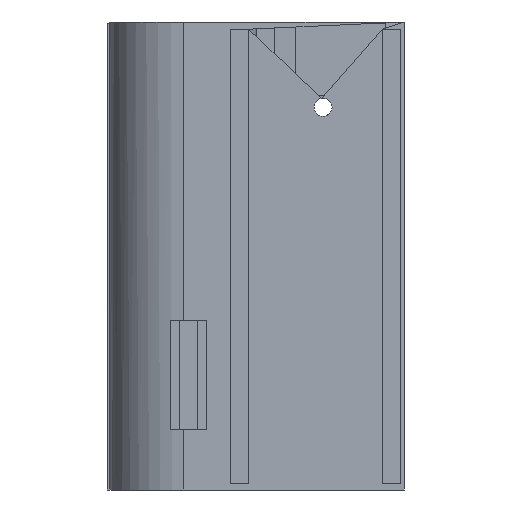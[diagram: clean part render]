
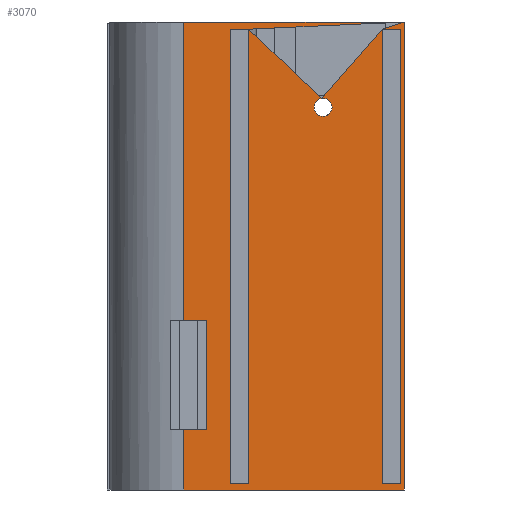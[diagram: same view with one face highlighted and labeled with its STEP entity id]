
A CAD part, left-side view. The second image highlights one B-rep face of the part: STEP entity #3070.
In plain terms, the highlighted planar face has unit normal (-1, 0, 0).
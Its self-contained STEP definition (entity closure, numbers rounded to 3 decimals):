
#5 = DIRECTION ( 'NONE',  ( 0., 0., -1. ) ) ;
#23 = ORIENTED_EDGE ( 'NONE', *, *, #3715, .T. ) ;
#29 = EDGE_CURVE ( 'NONE', #139, #4762, #4374, .T. ) ;
#71 = AXIS2_PLACEMENT_3D ( 'NONE', #1782, #1324, #1346 ) ;
#129 = LINE ( 'NONE', #1166, #960 ) ;
#139 = VERTEX_POINT ( 'NONE', #4965 ) ;
#177 = EDGE_LOOP ( 'NONE', ( #330, #702, #4123, #989 ) ) ;
#210 = EDGE_CURVE ( 'NONE', #4336, #4336, #4398, .T. ) ;
#241 = EDGE_CURVE ( 'NONE', #5273, #1962, #3889, .T. ) ;
#316 = VECTOR ( 'NONE', #2733, 1000. ) ;
#322 = CARTESIAN_POINT ( 'NONE',  ( -13., 25.767, -1. ) ) ;
#330 = ORIENTED_EDGE ( 'NONE', *, *, #569, .T. ) ;
#339 = CARTESIAN_POINT ( 'NONE',  ( -13., -10.668, 76.189 ) ) ;
#361 = DIRECTION ( 'NONE',  ( 0., -1., 0. ) ) ;
#369 = EDGE_CURVE ( 'NONE', #4762, #3531, #3568, .T. ) ;
#400 = EDGE_CURVE ( 'NONE', #467, #139, #3026, .T. ) ;
#467 = VERTEX_POINT ( 'NONE', #1895 ) ;
#504 = FACE_BOUND ( 'NONE', #1764, .T. ) ;
#536 = EDGE_CURVE ( 'NONE', #4986, #589, #129, .T. ) ;
#569 = EDGE_CURVE ( 'NONE', #2528, #1590, #4109, .T. ) ;
#589 = VERTEX_POINT ( 'NONE', #339 ) ;
#626 = DIRECTION ( 'NONE',  ( 0., 1., 0. ) ) ;
#669 = CARTESIAN_POINT ( 'NONE',  ( -13., -10.668, -1. ) ) ;
#702 = ORIENTED_EDGE ( 'NONE', *, *, #4699, .T. ) ;
#758 = CARTESIAN_POINT ( 'NONE',  ( -13., 25.767, 76.189 ) ) ;
#786 = CARTESIAN_POINT ( 'NONE',  ( -13., -10., 0. ) ) ;
#866 = CARTESIAN_POINT ( 'NONE',  ( -13., 21.9, 9. ) ) ;
#931 = CARTESIAN_POINT ( 'NONE',  ( -13., 21.9, 9. ) ) ;
#960 = VECTOR ( 'NONE', #1559, 1000. ) ;
#989 = ORIENTED_EDGE ( 'NONE', *, *, #3333, .T. ) ;
#1023 = VERTEX_POINT ( 'NONE', #758 ) ;
#1067 = VECTOR ( 'NONE', #1955, 1000. ) ;
#1096 = EDGE_LOOP ( 'NONE', ( #4860, #1400, #1157, #2286, #1209, #4950, #2393, #23 ) ) ;
#1124 = CARTESIAN_POINT ( 'NONE',  ( -13., 25.767, -1. ) ) ;
#1134 = CARTESIAN_POINT ( 'NONE',  ( -13., 25.767, -1. ) ) ;
#1154 = CARTESIAN_POINT ( 'NONE',  ( -13., 27.9, 27. ) ) ;
#1157 = ORIENTED_EDGE ( 'NONE', *, *, #3190, .T. ) ;
#1166 = CARTESIAN_POINT ( 'NONE',  ( -13., -10.668, -1. ) ) ;
#1205 = FACE_BOUND ( 'NONE', #177, .T. ) ;
#1209 = ORIENTED_EDGE ( 'NONE', *, *, #5067, .F. ) ;
#1219 = VECTOR ( 'NONE', #2648, 1000. ) ;
#1324 = DIRECTION ( 'NONE',  ( 1., 0., 0. ) ) ;
#1342 = PLANE ( 'NONE',  #2740 ) ;
#1346 = DIRECTION ( 'NONE',  ( 0., 1., 0. ) ) ;
#1400 = ORIENTED_EDGE ( 'NONE', *, *, #3306, .T. ) ;
#1415 = CARTESIAN_POINT ( 'NONE',  ( -13., 21.9, 27. ) ) ;
#1431 = VERTEX_POINT ( 'NONE', #322 ) ;
#1435 = CARTESIAN_POINT ( 'NONE',  ( -13., 18., 75. ) ) ;
#1449 = LINE ( 'NONE', #2551, #4335 ) ;
#1476 = EDGE_LOOP ( 'NONE', ( #4700, #1900, #1536, #1498 ) ) ;
#1490 = VERTEX_POINT ( 'NONE', #3621 ) ;
#1493 = VERTEX_POINT ( 'NONE', #2443 ) ;
#1498 = ORIENTED_EDGE ( 'NONE', *, *, #5166, .T. ) ;
#1505 = ORIENTED_EDGE ( 'NONE', *, *, #210, .T. ) ;
#1511 = EDGE_CURVE ( 'NONE', #1639, #1493, #5157, .T. ) ;
#1536 = ORIENTED_EDGE ( 'NONE', *, *, #369, .T. ) ;
#1559 = DIRECTION ( 'NONE',  ( 0., 0., 1. ) ) ;
#1590 = VERTEX_POINT ( 'NONE', #3296 ) ;
#1639 = VERTEX_POINT ( 'NONE', #4127 ) ;
#1708 = VECTOR ( 'NONE', #4285, 1000. ) ;
#1764 = EDGE_LOOP ( 'NONE', ( #1505 ) ) ;
#1782 = CARTESIAN_POINT ( 'NONE',  ( -13., 2.757, 62.126 ) ) ;
#1864 = VECTOR ( 'NONE', #4481, 1000. ) ;
#1895 = CARTESIAN_POINT ( 'NONE',  ( -13., 15., 0. ) ) ;
#1900 = ORIENTED_EDGE ( 'NONE', *, *, #29, .T. ) ;
#1955 = DIRECTION ( 'NONE',  ( 0., 0., 1. ) ) ;
#1962 = VERTEX_POINT ( 'NONE', #2776 ) ;
#2050 = LINE ( 'NONE', #1154, #1864 ) ;
#2109 = LINE ( 'NONE', #3135, #2825 ) ;
#2285 = CARTESIAN_POINT ( 'NONE',  ( -13., 15., 0. ) ) ;
#2286 = ORIENTED_EDGE ( 'NONE', *, *, #241, .T. ) ;
#2292 = LINE ( 'NONE', #4842, #4209 ) ;
#2372 = LINE ( 'NONE', #786, #2635 ) ;
#2380 = CARTESIAN_POINT ( 'NONE',  ( -13., 18., 0. ) ) ;
#2393 = ORIENTED_EDGE ( 'NONE', *, *, #536, .T. ) ;
#2414 = CARTESIAN_POINT ( 'NONE',  ( -13., 45.608, -1. ) ) ;
#2430 = LINE ( 'NONE', #2414, #2834 ) ;
#2443 = CARTESIAN_POINT ( 'NONE',  ( -13., -10., 0. ) ) ;
#2499 = DIRECTION ( 'NONE',  ( 0., -1., 0. ) ) ;
#2528 = VERTEX_POINT ( 'NONE', #4625 ) ;
#2551 = CARTESIAN_POINT ( 'NONE',  ( -13., -7., 75. ) ) ;
#2635 = VECTOR ( 'NONE', #4028, 1000. ) ;
#2648 = DIRECTION ( 'NONE',  ( 0., 1., 0. ) ) ;
#2698 = VECTOR ( 'NONE', #3248, 1000. ) ;
#2733 = DIRECTION ( 'NONE',  ( 0., 0., -1. ) ) ;
#2740 = AXIS2_PLACEMENT_3D ( 'NONE', #3395, #3783, #4595 ) ;
#2776 = CARTESIAN_POINT ( 'NONE',  ( -13., 25.767, 9. ) ) ;
#2825 = VECTOR ( 'NONE', #626, 1000. ) ;
#2834 = VECTOR ( 'NONE', #361, 1000. ) ;
#2890 = VECTOR ( 'NONE', #3910, 1000. ) ;
#2907 = LINE ( 'NONE', #1415, #5278 ) ;
#2914 = EDGE_CURVE ( 'NONE', #1023, #1490, #4107, .T. ) ;
#3026 = LINE ( 'NONE', #2285, #1219 ) ;
#3070 = ADVANCED_FACE ( 'NONE', ( #3658, #4849, #1205, #504 ), #1342, .T. ) ;
#3135 = CARTESIAN_POINT ( 'NONE',  ( -13., 15.471, 76.189 ) ) ;
#3190 = EDGE_CURVE ( 'NONE', #4493, #5273, #2907, .T. ) ;
#3213 = DIRECTION ( 'NONE',  ( 0., 0., 1. ) ) ;
#3232 = VECTOR ( 'NONE', #3213, 1000. ) ;
#3248 = DIRECTION ( 'NONE',  ( 0., 0., -1. ) ) ;
#3296 = CARTESIAN_POINT ( 'NONE',  ( -13., -7., 75. ) ) ;
#3297 = VECTOR ( 'NONE', #4428, 1000. ) ;
#3306 = EDGE_CURVE ( 'NONE', #1490, #4493, #2050, .T. ) ;
#3315 = EDGE_CURVE ( 'NONE', #1431, #4986, #2430, .T. ) ;
#3333 = EDGE_CURVE ( 'NONE', #1493, #2528, #2372, .T. ) ;
#3395 = CARTESIAN_POINT ( 'NONE',  ( -13., -10.668, -1. ) ) ;
#3450 = CARTESIAN_POINT ( 'NONE',  ( -13., 15., 75. ) ) ;
#3531 = VERTEX_POINT ( 'NONE', #3450 ) ;
#3568 = LINE ( 'NONE', #1435, #2890 ) ;
#3619 = CARTESIAN_POINT ( 'NONE',  ( -13., -7., 0. ) ) ;
#3621 = CARTESIAN_POINT ( 'NONE',  ( -13., 25.767, 27. ) ) ;
#3658 = FACE_BOUND ( 'NONE', #1476, .T. ) ;
#3700 = LINE ( 'NONE', #1124, #1067 ) ;
#3715 = EDGE_CURVE ( 'NONE', #589, #1023, #2109, .T. ) ;
#3783 = DIRECTION ( 'NONE',  ( -1., 0., 0. ) ) ;
#3813 = CARTESIAN_POINT ( 'NONE',  ( -13., 18., 75. ) ) ;
#3889 = LINE ( 'NONE', #931, #1708 ) ;
#3910 = DIRECTION ( 'NONE',  ( 0., -1., 0. ) ) ;
#4028 = DIRECTION ( 'NONE',  ( 0., 1., 0. ) ) ;
#4107 = LINE ( 'NONE', #1134, #316 ) ;
#4109 = LINE ( 'NONE', #3619, #3232 ) ;
#4123 = ORIENTED_EDGE ( 'NONE', *, *, #1511, .T. ) ;
#4127 = CARTESIAN_POINT ( 'NONE',  ( -13., -10., 75. ) ) ;
#4209 = VECTOR ( 'NONE', #5, 1000. ) ;
#4282 = DIRECTION ( 'NONE',  ( 0., 0., -1. ) ) ;
#4285 = DIRECTION ( 'NONE',  ( 0., 1., 0. ) ) ;
#4335 = VECTOR ( 'NONE', #2499, 1000. ) ;
#4336 = VERTEX_POINT ( 'NONE', #4553 ) ;
#4374 = LINE ( 'NONE', #2380, #3297 ) ;
#4398 = CIRCLE ( 'NONE', #71, 1.484 ) ;
#4428 = DIRECTION ( 'NONE',  ( 0., 0., 1. ) ) ;
#4481 = DIRECTION ( 'NONE',  ( 0., -1., 0. ) ) ;
#4493 = VERTEX_POINT ( 'NONE', #4863 ) ;
#4494 = CARTESIAN_POINT ( 'NONE',  ( -13., -10., 75. ) ) ;
#4553 = CARTESIAN_POINT ( 'NONE',  ( -13., 4.241, 62.126 ) ) ;
#4595 = DIRECTION ( 'NONE',  ( 0., 1., 0. ) ) ;
#4625 = CARTESIAN_POINT ( 'NONE',  ( -13., -7., 0. ) ) ;
#4699 = EDGE_CURVE ( 'NONE', #1590, #1639, #1449, .T. ) ;
#4700 = ORIENTED_EDGE ( 'NONE', *, *, #400, .T. ) ;
#4762 = VERTEX_POINT ( 'NONE', #3813 ) ;
#4842 = CARTESIAN_POINT ( 'NONE',  ( -13., 15., 75. ) ) ;
#4849 = FACE_OUTER_BOUND ( 'NONE', #1096, .T. ) ;
#4860 = ORIENTED_EDGE ( 'NONE', *, *, #2914, .T. ) ;
#4863 = CARTESIAN_POINT ( 'NONE',  ( -13., 21.9, 27. ) ) ;
#4950 = ORIENTED_EDGE ( 'NONE', *, *, #3315, .T. ) ;
#4965 = CARTESIAN_POINT ( 'NONE',  ( -13., 18., 0. ) ) ;
#4986 = VERTEX_POINT ( 'NONE', #669 ) ;
#5067 = EDGE_CURVE ( 'NONE', #1431, #1962, #3700, .T. ) ;
#5157 = LINE ( 'NONE', #4494, #2698 ) ;
#5166 = EDGE_CURVE ( 'NONE', #3531, #467, #2292, .T. ) ;
#5273 = VERTEX_POINT ( 'NONE', #866 ) ;
#5278 = VECTOR ( 'NONE', #4282, 1000. ) ;
